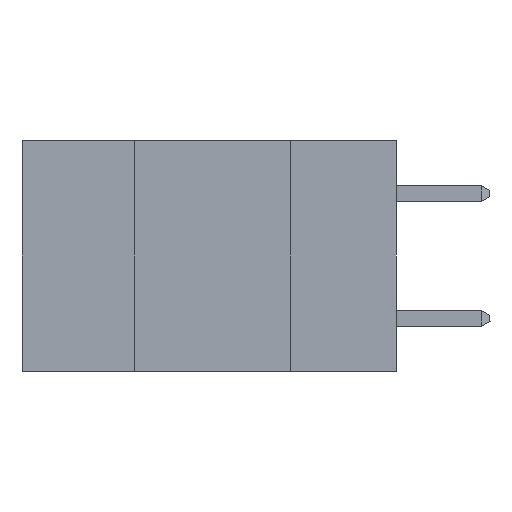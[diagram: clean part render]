
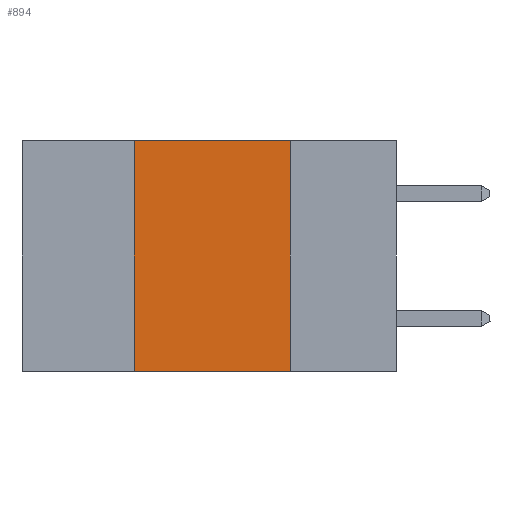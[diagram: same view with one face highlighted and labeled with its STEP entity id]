
A CAD part, left-side view. The second image highlights one B-rep face of the part: STEP entity #894.
In plain terms, the highlighted planar face has unit normal (-1, 0, 0).
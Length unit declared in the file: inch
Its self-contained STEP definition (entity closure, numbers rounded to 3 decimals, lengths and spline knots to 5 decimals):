
#38 = VERTEX_POINT ( 'NONE', #7347 ) ;
#547 = ORIENTED_EDGE ( 'NONE', *, *, #8252, .F. ) ;
#894 = ADVANCED_FACE ( 'NONE', ( #4966 ), #13894, .F. ) ;
#935 = VERTEX_POINT ( 'NONE', #17846 ) ;
#1081 = VECTOR ( 'NONE', #19261, 39.37008 ) ;
#3256 = CARTESIAN_POINT ( 'NONE',  ( 0., 0.6, -0.37 ) ) ;
#4026 = DIRECTION ( 'NONE',  ( 0., -1., 0. ) ) ;
#4966 = FACE_OUTER_BOUND ( 'NONE', #20624, .T. ) ;
#5063 = VECTOR ( 'NONE', #16230, 39.37008 ) ;
#7347 = CARTESIAN_POINT ( 'NONE',  ( 0., 0.42, -0.37 ) ) ;
#7408 = AXIS2_PLACEMENT_3D ( 'NONE', #18576, #23572, #7686 ) ;
#7686 = DIRECTION ( 'NONE',  ( 0., 0., -1. ) ) ;
#8191 = ORIENTED_EDGE ( 'NONE', *, *, #19637, .F. ) ;
#8252 = EDGE_CURVE ( 'NONE', #38, #935, #16107, .T. ) ;
#9164 = LINE ( 'NONE', #17191, #18027 ) ;
#9281 = ORIENTED_EDGE ( 'NONE', *, *, #11666, .F. ) ;
#9376 = VERTEX_POINT ( 'NONE', #16151 ) ;
#9961 = VECTOR ( 'NONE', #18317, 39.37008 ) ;
#11666 = EDGE_CURVE ( 'NONE', #935, #21968, #9164, .T. ) ;
#13894 = PLANE ( 'NONE',  #7408 ) ;
#15078 = LINE ( 'NONE', #18042, #5063 ) ;
#15852 = EDGE_CURVE ( 'NONE', #38, #9376, #19995, .T. ) ;
#16107 = LINE ( 'NONE', #21067, #1081 ) ;
#16151 = CARTESIAN_POINT ( 'NONE',  ( 0., 0.17, -0.37 ) ) ;
#16230 = DIRECTION ( 'NONE',  ( 0., 0., -1. ) ) ;
#17191 = CARTESIAN_POINT ( 'NONE',  ( 0., 0.6, 0. ) ) ;
#17846 = CARTESIAN_POINT ( 'NONE',  ( 0., 0.42, 0. ) ) ;
#18027 = VECTOR ( 'NONE', #4026, 39.37008 ) ;
#18042 = CARTESIAN_POINT ( 'NONE',  ( 0., 0.17, 0. ) ) ;
#18317 = DIRECTION ( 'NONE',  ( 0., -1., 0. ) ) ;
#18576 = CARTESIAN_POINT ( 'NONE',  ( 0., 0.6, 0. ) ) ;
#19261 = DIRECTION ( 'NONE',  ( 0., 0., 1. ) ) ;
#19637 = EDGE_CURVE ( 'NONE', #21968, #9376, #15078, .T. ) ;
#19995 = LINE ( 'NONE', #3256, #9961 ) ;
#20624 = EDGE_LOOP ( 'NONE', ( #8191, #9281, #547, #21744 ) ) ;
#21067 = CARTESIAN_POINT ( 'NONE',  ( 0., 0.42, 0. ) ) ;
#21744 = ORIENTED_EDGE ( 'NONE', *, *, #15852, .T. ) ;
#21968 = VERTEX_POINT ( 'NONE', #22842 ) ;
#22842 = CARTESIAN_POINT ( 'NONE',  ( 0., 0.17, 0. ) ) ;
#23572 = DIRECTION ( 'NONE',  ( 1., 0., 0. ) ) ;
